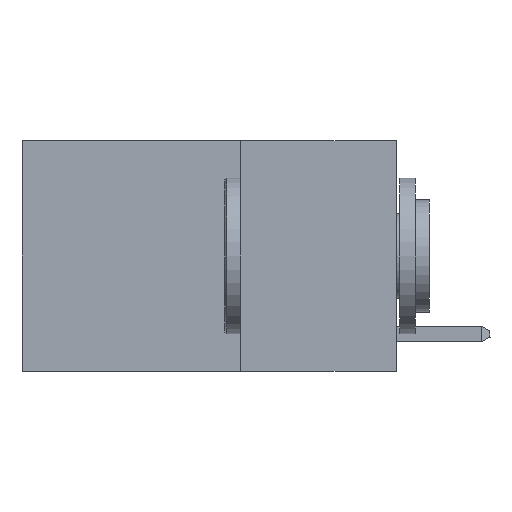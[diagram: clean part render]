
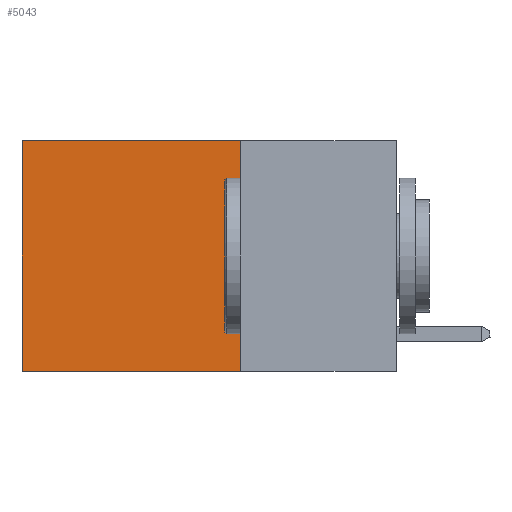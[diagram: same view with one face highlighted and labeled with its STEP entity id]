
A CAD part, left-side view. The second image highlights one B-rep face of the part: STEP entity #5043.
In plain terms, the highlighted planar face has unit normal (-1, 0, 0).
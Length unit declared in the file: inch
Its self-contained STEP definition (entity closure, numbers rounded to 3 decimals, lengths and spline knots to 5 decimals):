
#179 = LINE ( 'NONE', #2245, #5948 ) ;
#363 = DIRECTION ( 'NONE',  ( 0., 1., 0. ) ) ;
#519 = AXIS2_PLACEMENT_3D ( 'NONE', #7468, #4534, #9683 ) ;
#740 = DIRECTION ( 'NONE',  ( 0., 0., -1. ) ) ;
#974 = DIRECTION ( 'NONE',  ( 0., 1., 0. ) ) ;
#1367 = VECTOR ( 'NONE', #363, 39.37008 ) ;
#2072 = ORIENTED_EDGE ( 'NONE', *, *, #6991, .T. ) ;
#2245 = CARTESIAN_POINT ( 'NONE',  ( 0.2625, 0.25, 0. ) ) ;
#2932 = EDGE_LOOP ( 'NONE', ( #5767, #7772, #9706, #2072 ) ) ;
#3186 = VECTOR ( 'NONE', #740, 39.37008 ) ;
#3306 = CARTESIAN_POINT ( 'NONE',  ( 0.2625, 0.6, -0.37 ) ) ;
#3495 = EDGE_CURVE ( 'NONE', #8789, #6935, #5139, .T. ) ;
#3678 = CARTESIAN_POINT ( 'NONE',  ( 0.2625, 0.25, -0.37 ) ) ;
#4423 = CARTESIAN_POINT ( 'NONE',  ( 0.2625, 0.6, 0. ) ) ;
#4534 = DIRECTION ( 'NONE',  ( 1., 0., 0. ) ) ;
#5043 = ADVANCED_FACE ( 'NONE', ( #8830 ), #8969, .F. ) ;
#5139 = LINE ( 'NONE', #4423, #3186 ) ;
#5416 = CARTESIAN_POINT ( 'NONE',  ( 0.2625, 0.25, -0.37 ) ) ;
#5511 = LINE ( 'NONE', #5416, #9668 ) ;
#5623 = CARTESIAN_POINT ( 'NONE',  ( 0.2625, 0.25, 0. ) ) ;
#5767 = ORIENTED_EDGE ( 'NONE', *, *, #3495, .T. ) ;
#5948 = VECTOR ( 'NONE', #8191, 39.37008 ) ;
#6508 = VERTEX_POINT ( 'NONE', #3678 ) ;
#6935 = VERTEX_POINT ( 'NONE', #3306 ) ;
#6991 = EDGE_CURVE ( 'NONE', #9612, #8789, #7511, .T. ) ;
#7468 = CARTESIAN_POINT ( 'NONE',  ( 0.2625, 0.25, 0. ) ) ;
#7511 = LINE ( 'NONE', #8596, #1367 ) ;
#7730 = CARTESIAN_POINT ( 'NONE',  ( 0.2625, 0.6, 0. ) ) ;
#7772 = ORIENTED_EDGE ( 'NONE', *, *, #8070, .F. ) ;
#8070 = EDGE_CURVE ( 'NONE', #6508, #6935, #5511, .T. ) ;
#8191 = DIRECTION ( 'NONE',  ( 0., 0., -1. ) ) ;
#8482 = EDGE_CURVE ( 'NONE', #9612, #6508, #179, .T. ) ;
#8596 = CARTESIAN_POINT ( 'NONE',  ( 0.2625, 0.25, 0. ) ) ;
#8789 = VERTEX_POINT ( 'NONE', #7730 ) ;
#8830 = FACE_OUTER_BOUND ( 'NONE', #2932, .T. ) ;
#8969 = PLANE ( 'NONE',  #519 ) ;
#9612 = VERTEX_POINT ( 'NONE', #5623 ) ;
#9668 = VECTOR ( 'NONE', #974, 39.37008 ) ;
#9683 = DIRECTION ( 'NONE',  ( 0., 0., -1. ) ) ;
#9706 = ORIENTED_EDGE ( 'NONE', *, *, #8482, .F. ) ;
